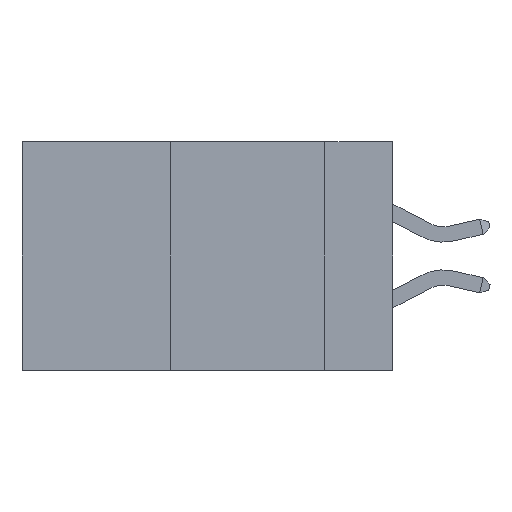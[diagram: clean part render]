
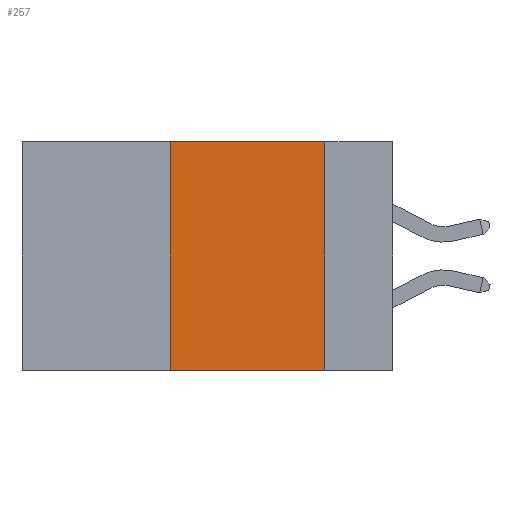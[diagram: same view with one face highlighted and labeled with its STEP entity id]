
A CAD part, left-side view. The second image highlights one B-rep face of the part: STEP entity #257.
In plain terms, the highlighted planar face has unit normal (-1, 0, 0).
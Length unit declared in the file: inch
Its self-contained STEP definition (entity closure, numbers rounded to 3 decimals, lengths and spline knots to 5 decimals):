
#257 = ADVANCED_FACE ( 'NONE', ( #11641 ), #2695, .F. ) ;
#269 = CARTESIAN_POINT ( 'NONE',  ( 0., 0.11, 0. ) ) ;
#478 = CARTESIAN_POINT ( 'NONE',  ( 0., 0.11, -0.37 ) ) ;
#1308 = ORIENTED_EDGE ( 'NONE', *, *, #11687, .T. ) ;
#1345 = LINE ( 'NONE', #8708, #5493 ) ;
#1902 = DIRECTION ( 'NONE',  ( 1., 0., 0. ) ) ;
#2504 = ORIENTED_EDGE ( 'NONE', *, *, #7467, .F. ) ;
#2695 = PLANE ( 'NONE',  #5819 ) ;
#2726 = CARTESIAN_POINT ( 'NONE',  ( 0., 0.36, -0.37 ) ) ;
#2831 = DIRECTION ( 'NONE',  ( 0., -1., 0. ) ) ;
#2901 = LINE ( 'NONE', #3115, #7493 ) ;
#3115 = CARTESIAN_POINT ( 'NONE',  ( 0., 0.6, 0. ) ) ;
#3141 = ORIENTED_EDGE ( 'NONE', *, *, #8804, .F. ) ;
#3581 = DIRECTION ( 'NONE',  ( 0., 0., 1. ) ) ;
#3863 = VERTEX_POINT ( 'NONE', #478 ) ;
#4258 = VECTOR ( 'NONE', #2831, 39.37008 ) ;
#4566 = CARTESIAN_POINT ( 'NONE',  ( 0., 0.6, 0. ) ) ;
#5398 = LINE ( 'NONE', #10315, #4258 ) ;
#5487 = VERTEX_POINT ( 'NONE', #269 ) ;
#5493 = VECTOR ( 'NONE', #9722, 39.37008 ) ;
#5819 = AXIS2_PLACEMENT_3D ( 'NONE', #4566, #1902, #10057 ) ;
#6847 = DIRECTION ( 'NONE',  ( 0., -1., 0. ) ) ;
#6926 = EDGE_CURVE ( 'NONE', #5487, #3863, #1345, .T. ) ;
#7184 = ORIENTED_EDGE ( 'NONE', *, *, #6926, .F. ) ;
#7219 = VERTEX_POINT ( 'NONE', #9180 ) ;
#7467 = EDGE_CURVE ( 'NONE', #7219, #5487, #2901, .T. ) ;
#7493 = VECTOR ( 'NONE', #6847, 39.37008 ) ;
#7811 = VERTEX_POINT ( 'NONE', #2726 ) ;
#8182 = CARTESIAN_POINT ( 'NONE',  ( 0., 0.36, 0. ) ) ;
#8708 = CARTESIAN_POINT ( 'NONE',  ( 0., 0.11, 0. ) ) ;
#8804 = EDGE_CURVE ( 'NONE', #7811, #7219, #10489, .T. ) ;
#9180 = CARTESIAN_POINT ( 'NONE',  ( 0., 0.36, 0. ) ) ;
#9722 = DIRECTION ( 'NONE',  ( 0., 0., -1. ) ) ;
#10056 = VECTOR ( 'NONE', #3581, 39.37008 ) ;
#10057 = DIRECTION ( 'NONE',  ( 0., 0., -1. ) ) ;
#10315 = CARTESIAN_POINT ( 'NONE',  ( 0., 0.6, -0.37 ) ) ;
#10489 = LINE ( 'NONE', #8182, #10056 ) ;
#11400 = EDGE_LOOP ( 'NONE', ( #7184, #2504, #3141, #1308 ) ) ;
#11641 = FACE_OUTER_BOUND ( 'NONE', #11400, .T. ) ;
#11687 = EDGE_CURVE ( 'NONE', #7811, #3863, #5398, .T. ) ;
